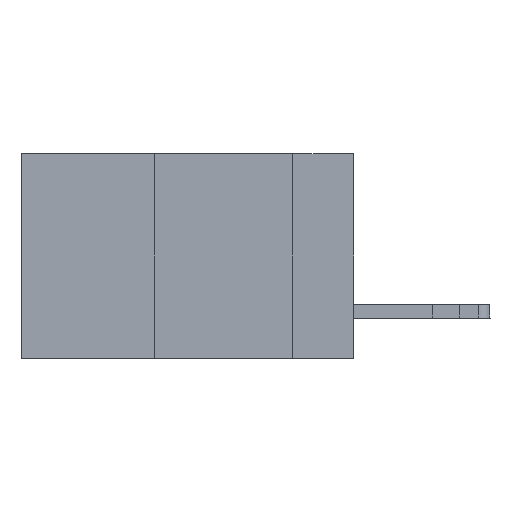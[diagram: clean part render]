
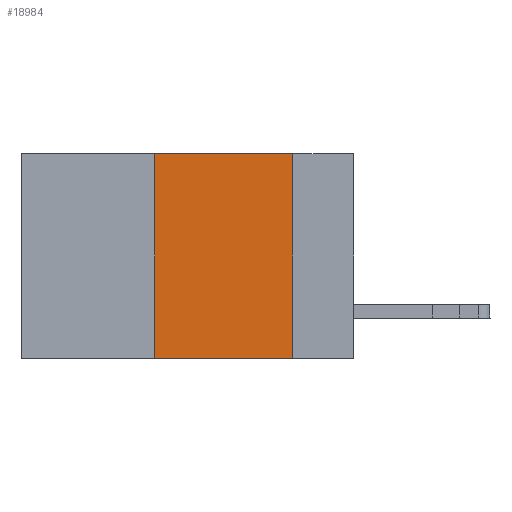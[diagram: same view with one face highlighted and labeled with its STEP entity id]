
A CAD part, left-side view. The second image highlights one B-rep face of the part: STEP entity #18984.
In plain terms, the highlighted planar face has unit normal (-1, 0, 0).
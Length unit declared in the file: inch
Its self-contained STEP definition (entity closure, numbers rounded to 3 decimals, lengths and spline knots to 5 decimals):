
#274 = FACE_OUTER_BOUND ( 'NONE', #23494, .T. ) ;
#1583 = LINE ( 'NONE', #26602, #1932 ) ;
#1932 = VECTOR ( 'NONE', #26888, 39.37008 ) ;
#5050 = CARTESIAN_POINT ( 'NONE',  ( 0., 0.6, 0. ) ) ;
#6035 = AXIS2_PLACEMENT_3D ( 'NONE', #5050, #13984, #26609 ) ;
#6082 = LINE ( 'NONE', #10025, #10850 ) ;
#6225 = CARTESIAN_POINT ( 'NONE',  ( 0., 0.11, 0. ) ) ;
#7957 = CARTESIAN_POINT ( 'NONE',  ( 0., 0.6, -0.37 ) ) ;
#9691 = ORIENTED_EDGE ( 'NONE', *, *, #19596, .F. ) ;
#10025 = CARTESIAN_POINT ( 'NONE',  ( 0., 0.6, 0. ) ) ;
#10481 = DIRECTION ( 'NONE',  ( 0., -1., 0. ) ) ;
#10850 = VECTOR ( 'NONE', #10481, 39.37008 ) ;
#10927 = ORIENTED_EDGE ( 'NONE', *, *, #16516, .F. ) ;
#12951 = VECTOR ( 'NONE', #20728, 39.37008 ) ;
#13367 = ORIENTED_EDGE ( 'NONE', *, *, #25993, .F. ) ;
#13984 = DIRECTION ( 'NONE',  ( 1., 0., 0. ) ) ;
#14783 = EDGE_CURVE ( 'NONE', #23562, #20994, #26438, .T. ) ;
#15107 = CARTESIAN_POINT ( 'NONE',  ( 0., 0.11, -0.37 ) ) ;
#16516 = EDGE_CURVE ( 'NONE', #20116, #22595, #6082, .T. ) ;
#18984 = ADVANCED_FACE ( 'NONE', ( #274 ), #24143, .F. ) ;
#19288 = CARTESIAN_POINT ( 'NONE',  ( 0., 0.36, -0.37 ) ) ;
#19596 = EDGE_CURVE ( 'NONE', #23562, #20116, #1583, .T. ) ;
#19834 = VECTOR ( 'NONE', #26135, 39.37008 ) ;
#20116 = VERTEX_POINT ( 'NONE', #23159 ) ;
#20728 = DIRECTION ( 'NONE',  ( 0., -1., 0. ) ) ;
#20994 = VERTEX_POINT ( 'NONE', #15107 ) ;
#22595 = VERTEX_POINT ( 'NONE', #6225 ) ;
#23159 = CARTESIAN_POINT ( 'NONE',  ( 0., 0.36, 0. ) ) ;
#23494 = EDGE_LOOP ( 'NONE', ( #13367, #10927, #9691, #25017 ) ) ;
#23562 = VERTEX_POINT ( 'NONE', #19288 ) ;
#23852 = CARTESIAN_POINT ( 'NONE',  ( 0., 0.11, 0. ) ) ;
#24143 = PLANE ( 'NONE',  #6035 ) ;
#25017 = ORIENTED_EDGE ( 'NONE', *, *, #14783, .T. ) ;
#25993 = EDGE_CURVE ( 'NONE', #22595, #20994, #26937, .T. ) ;
#26135 = DIRECTION ( 'NONE',  ( 0., 0., -1. ) ) ;
#26438 = LINE ( 'NONE', #7957, #12951 ) ;
#26602 = CARTESIAN_POINT ( 'NONE',  ( 0., 0.36, 0. ) ) ;
#26609 = DIRECTION ( 'NONE',  ( 0., 0., -1. ) ) ;
#26888 = DIRECTION ( 'NONE',  ( 0., 0., 1. ) ) ;
#26937 = LINE ( 'NONE', #23852, #19834 ) ;
